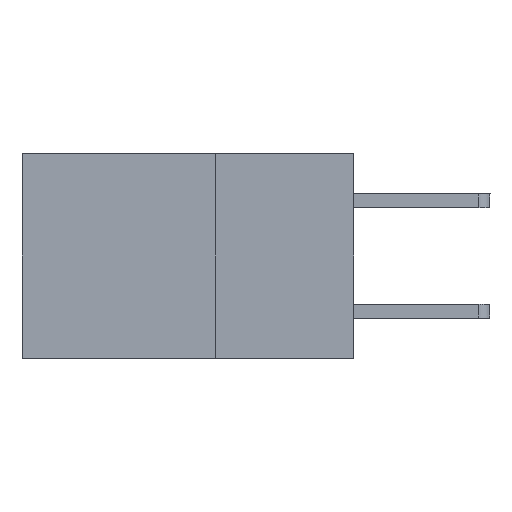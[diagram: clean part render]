
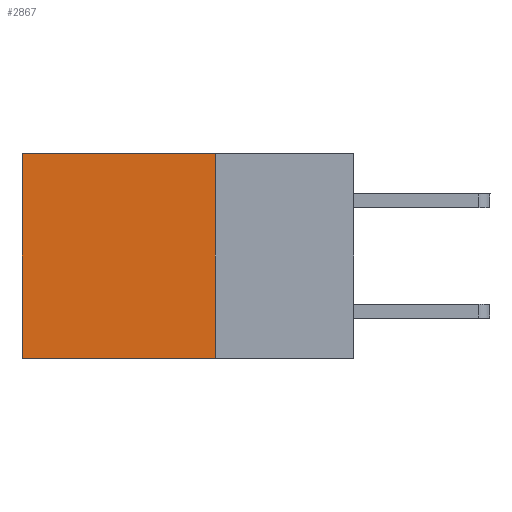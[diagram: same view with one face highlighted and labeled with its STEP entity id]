
A CAD part, left-side view. The second image highlights one B-rep face of the part: STEP entity #2867.
In plain terms, the highlighted planar face has unit normal (-1, 0, 0).
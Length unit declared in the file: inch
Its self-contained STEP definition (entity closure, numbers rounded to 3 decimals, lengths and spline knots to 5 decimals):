
#12 = CARTESIAN_POINT ( 'NONE',  ( 0.2875, 0.6, 0. ) ) ;
#243 = VERTEX_POINT ( 'NONE', #12 ) ;
#611 = VECTOR ( 'NONE', #8942, 39.37008 ) ;
#1987 = AXIS2_PLACEMENT_3D ( 'NONE', #9484, #9460, #9445 ) ;
#2637 = ORIENTED_EDGE ( 'NONE', *, *, #6676, .T. ) ;
#2649 = ORIENTED_EDGE ( 'NONE', *, *, #8546, .F. ) ;
#2706 = LINE ( 'NONE', #8613, #11919 ) ;
#2867 = ADVANCED_FACE ( 'NONE', ( #5971 ), #9547, .F. ) ;
#2889 = EDGE_CURVE ( 'NONE', #243, #9903, #2976, .T. ) ;
#2976 = LINE ( 'NONE', #8956, #611 ) ;
#3449 = DIRECTION ( 'NONE',  ( 0., 1., 0. ) ) ;
#3608 = VERTEX_POINT ( 'NONE', #9526 ) ;
#4528 = CARTESIAN_POINT ( 'NONE',  ( 0.2875, 0.6, -0.37 ) ) ;
#5118 = ORIENTED_EDGE ( 'NONE', *, *, #2889, .T. ) ;
#5152 = CARTESIAN_POINT ( 'NONE',  ( 0.2875, 0.25, 0. ) ) ;
#5541 = LINE ( 'NONE', #5152, #9958 ) ;
#5971 = FACE_OUTER_BOUND ( 'NONE', #11626, .T. ) ;
#5989 = DIRECTION ( 'NONE',  ( 0., 1., 0. ) ) ;
#6351 = CARTESIAN_POINT ( 'NONE',  ( 0.2875, 0.25, -0.37 ) ) ;
#6676 = EDGE_CURVE ( 'NONE', #3608, #243, #2706, .T. ) ;
#8312 = VERTEX_POINT ( 'NONE', #9359 ) ;
#8546 = EDGE_CURVE ( 'NONE', #3608, #8312, #5541, .T. ) ;
#8613 = CARTESIAN_POINT ( 'NONE',  ( 0.2875, 0.25, 0. ) ) ;
#8929 = EDGE_CURVE ( 'NONE', #8312, #9903, #9529, .T. ) ;
#8942 = DIRECTION ( 'NONE',  ( 0., 0., -1. ) ) ;
#8956 = CARTESIAN_POINT ( 'NONE',  ( 0.2875, 0.6, 0. ) ) ;
#9359 = CARTESIAN_POINT ( 'NONE',  ( 0.2875, 0.25, -0.37 ) ) ;
#9445 = DIRECTION ( 'NONE',  ( 0., 0., -1. ) ) ;
#9460 = DIRECTION ( 'NONE',  ( 1., 0., 0. ) ) ;
#9484 = CARTESIAN_POINT ( 'NONE',  ( 0.2875, 0.25, 0. ) ) ;
#9526 = CARTESIAN_POINT ( 'NONE',  ( 0.2875, 0.25, 0. ) ) ;
#9529 = LINE ( 'NONE', #6351, #11860 ) ;
#9547 = PLANE ( 'NONE',  #1987 ) ;
#9830 = ORIENTED_EDGE ( 'NONE', *, *, #8929, .F. ) ;
#9903 = VERTEX_POINT ( 'NONE', #4528 ) ;
#9958 = VECTOR ( 'NONE', #11298, 39.37008 ) ;
#11298 = DIRECTION ( 'NONE',  ( 0., 0., -1. ) ) ;
#11626 = EDGE_LOOP ( 'NONE', ( #5118, #9830, #2649, #2637 ) ) ;
#11860 = VECTOR ( 'NONE', #3449, 39.37008 ) ;
#11919 = VECTOR ( 'NONE', #5989, 39.37008 ) ;
